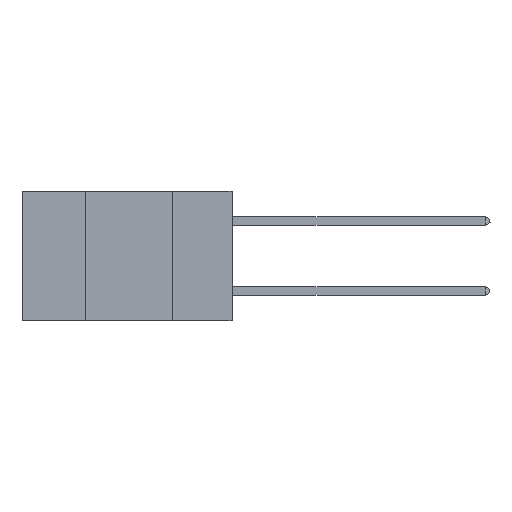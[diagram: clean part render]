
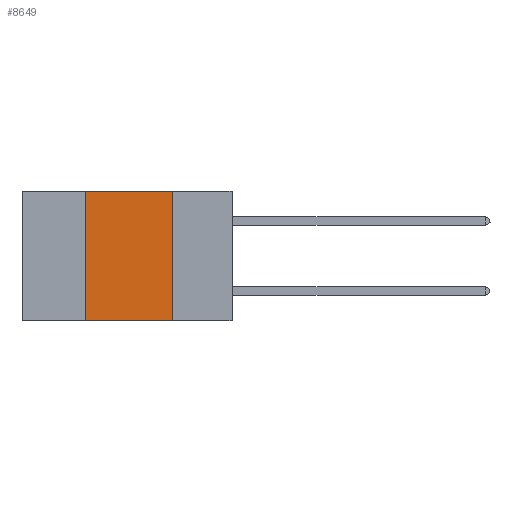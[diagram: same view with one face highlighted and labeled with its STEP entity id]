
A CAD part, left-side view. The second image highlights one B-rep face of the part: STEP entity #8649.
In plain terms, the highlighted planar face has unit normal (-1, 0, 0).
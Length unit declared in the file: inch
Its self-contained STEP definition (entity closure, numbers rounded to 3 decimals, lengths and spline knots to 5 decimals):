
#4188 = DIRECTION ( 'NONE',  ( 1., 0., 0. ) ) ;
#4494 = CARTESIAN_POINT ( 'NONE',  ( 0., 0.6, 0. ) ) ;
#5019 = VECTOR ( 'NONE', #23715, 39.37008 ) ;
#6857 = FACE_OUTER_BOUND ( 'NONE', #24547, .T. ) ;
#7421 = LINE ( 'NONE', #26346, #13236 ) ;
#8591 = ORIENTED_EDGE ( 'NONE', *, *, #9124, .F. ) ;
#8649 = ADVANCED_FACE ( 'NONE', ( #6857 ), #16096, .F. ) ;
#8961 = ORIENTED_EDGE ( 'NONE', *, *, #29551, .F. ) ;
#9124 = EDGE_CURVE ( 'NONE', #18755, #24218, #7421, .T. ) ;
#9517 = ORIENTED_EDGE ( 'NONE', *, *, #16534, .T. ) ;
#11393 = DIRECTION ( 'NONE',  ( 0., 0., -1. ) ) ;
#11567 = LINE ( 'NONE', #20644, #12009 ) ;
#12009 = VECTOR ( 'NONE', #16118, 39.37008 ) ;
#13236 = VECTOR ( 'NONE', #26800, 39.37008 ) ;
#13355 = CARTESIAN_POINT ( 'NONE',  ( 0., 0.17, -0.37 ) ) ;
#13641 = VERTEX_POINT ( 'NONE', #13355 ) ;
#14005 = CARTESIAN_POINT ( 'NONE',  ( 0., 0.42, 0. ) ) ;
#14322 = CARTESIAN_POINT ( 'NONE',  ( 0., 0.17, 0. ) ) ;
#16096 = PLANE ( 'NONE',  #20114 ) ;
#16118 = DIRECTION ( 'NONE',  ( 0., -1., 0. ) ) ;
#16534 = EDGE_CURVE ( 'NONE', #18755, #13641, #18703, .T. ) ;
#17736 = CARTESIAN_POINT ( 'NONE',  ( 0., 0.17, 0. ) ) ;
#17855 = EDGE_CURVE ( 'NONE', #25673, #13641, #26336, .T. ) ;
#18703 = LINE ( 'NONE', #30753, #25969 ) ;
#18755 = VERTEX_POINT ( 'NONE', #23182 ) ;
#20114 = AXIS2_PLACEMENT_3D ( 'NONE', #4494, #4188, #11393 ) ;
#20644 = CARTESIAN_POINT ( 'NONE',  ( 0., 0.6, 0. ) ) ;
#23182 = CARTESIAN_POINT ( 'NONE',  ( 0., 0.42, -0.37 ) ) ;
#23552 = DIRECTION ( 'NONE',  ( 0., -1., 0. ) ) ;
#23715 = DIRECTION ( 'NONE',  ( 0., 0., -1. ) ) ;
#24218 = VERTEX_POINT ( 'NONE', #14005 ) ;
#24547 = EDGE_LOOP ( 'NONE', ( #28448, #8961, #8591, #9517 ) ) ;
#25673 = VERTEX_POINT ( 'NONE', #17736 ) ;
#25969 = VECTOR ( 'NONE', #23552, 39.37008 ) ;
#26336 = LINE ( 'NONE', #14322, #5019 ) ;
#26346 = CARTESIAN_POINT ( 'NONE',  ( 0., 0.42, 0. ) ) ;
#26800 = DIRECTION ( 'NONE',  ( 0., 0., 1. ) ) ;
#28448 = ORIENTED_EDGE ( 'NONE', *, *, #17855, .F. ) ;
#29551 = EDGE_CURVE ( 'NONE', #24218, #25673, #11567, .T. ) ;
#30753 = CARTESIAN_POINT ( 'NONE',  ( 0., 0.6, -0.37 ) ) ;
